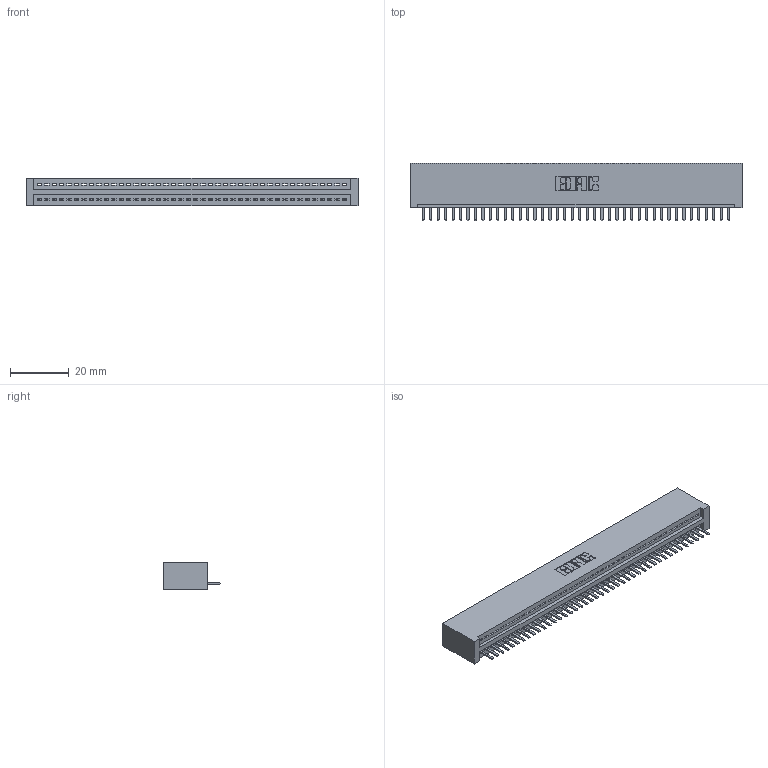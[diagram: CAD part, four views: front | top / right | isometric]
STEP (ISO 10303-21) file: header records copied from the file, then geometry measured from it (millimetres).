
FILE_DESCRIPTION (( 'STEP AP203' ), '1' );
FILE_NAME ('345-042-520-101.STEP', '2018-09-05T10:28:45', ( '' ), ( '' ), 'SwSTEP 2.0', 'SolidWorks 2016', '' );
FILE_SCHEMA (( 'CONFIG_CONTROL_DESIGN' ));
Length unit declared in the file: inch
Products named in the file (3): 345 Part_No Mounting Lugs; 345-292-001_345-293-120; 345-042-520-101
Assembly tree (43 placements, depth 2):
  345-042-520-101
    345 Part_No Mounting Lugs
    345-292-001_345-293-120  x42
Bounding box: 113.28 x 19.68 x 9.4 mm (x, y, z)
Volume: 11223.4 mm3; surface area: 14709.8 mm2
Topology: 43 solids, 43 shells, 2722 faces, 8045 edges, 5250 vertices
Faces by surface type: plane 1840, cylinder 882
Entity records: 31447 total; most frequent: CARTESIAN_POINT 5466, ORIENTED_EDGE 5430, DIRECTION 4755, EDGE_CURVE 2715, LINE 2419, VECTOR 2419, VERTEX_POINT 1806, AXIS2_PLACEMENT_3D 1168
